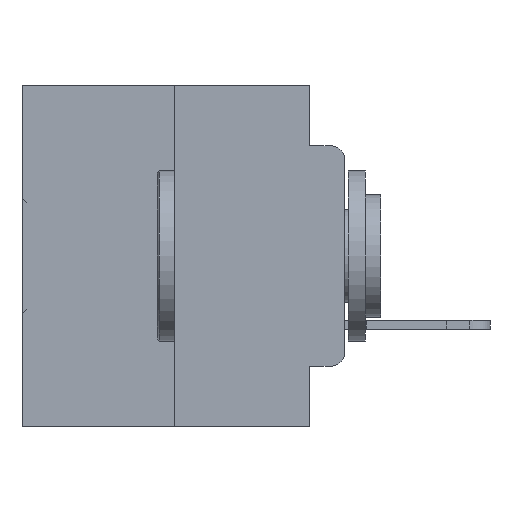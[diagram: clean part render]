
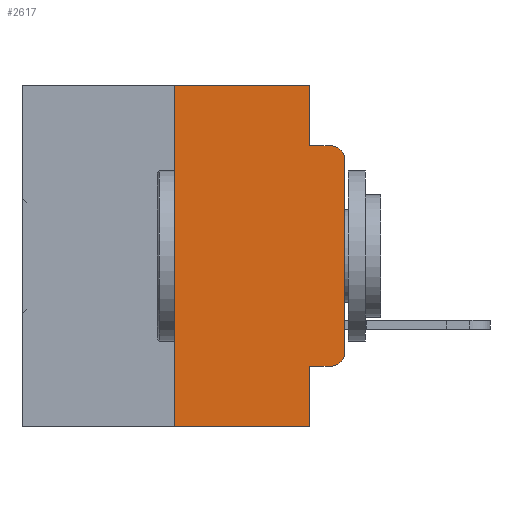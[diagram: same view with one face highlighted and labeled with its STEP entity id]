
A CAD part, left-side view. The second image highlights one B-rep face of the part: STEP entity #2617.
In plain terms, the highlighted planar face has unit normal (-1, 0, 0).
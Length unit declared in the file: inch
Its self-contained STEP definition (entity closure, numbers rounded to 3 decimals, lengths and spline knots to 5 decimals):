
#250 = ORIENTED_EDGE ( 'NONE', *, *, #6677, .T. ) ;
#1705 = CARTESIAN_POINT ( 'NONE',  ( 0., 0.051, -0.4115 ) ) ;
#1734 = ORIENTED_EDGE ( 'NONE', *, *, #12036, .F. ) ;
#1771 = LINE ( 'NONE', #17160, #15361 ) ;
#1961 = ORIENTED_EDGE ( 'NONE', *, *, #12135, .T. ) ;
#2097 = ORIENTED_EDGE ( 'NONE', *, *, #12140, .T. ) ;
#2617 = ADVANCED_FACE ( 'NONE', ( #4248 ), #13347, .F. ) ;
#4248 = FACE_OUTER_BOUND ( 'NONE', #5648, .T. ) ;
#5395 = VERTEX_POINT ( 'NONE', #32085 ) ;
#5648 = EDGE_LOOP ( 'NONE', ( #19901, #22186, #23280, #25613, #26177, #27823, #250, #1734, #1961, #2097 ) ) ;
#6668 = EDGE_CURVE ( 'NONE', #33246, #11114, #23879, .T. ) ;
#6677 = EDGE_CURVE ( 'NONE', #12878, #30754, #23019, .T. ) ;
#6907 = DIRECTION ( 'NONE',  ( 0., 0., -1. ) ) ;
#6994 = LINE ( 'NONE', #1705, #20261 ) ;
#7294 = CARTESIAN_POINT ( 'NONE',  ( 0., 0.02, -0.0885 ) ) ;
#7665 = CARTESIAN_POINT ( 'NONE',  ( 0., 0.051, 0. ) ) ;
#8056 = AXIS2_PLACEMENT_3D ( 'NONE', #18046, #33623, #17933 ) ;
#8332 = LINE ( 'NONE', #16361, #21516 ) ;
#9598 = VECTOR ( 'NONE', #6907, 39.37008 ) ;
#10053 = CIRCLE ( 'NONE', #8056, 0.02 ) ;
#10061 = VERTEX_POINT ( 'NONE', #12943 ) ;
#10124 = VERTEX_POINT ( 'NONE', #7294 ) ;
#10225 = DIRECTION ( 'NONE',  ( 0., 0., 1. ) ) ;
#11114 = VERTEX_POINT ( 'NONE', #12263 ) ;
#11682 = VECTOR ( 'NONE', #22231, 39.37008 ) ;
#11764 = EDGE_CURVE ( 'NONE', #33010, #33686, #32170, .T. ) ;
#11826 = EDGE_CURVE ( 'NONE', #33686, #10124, #10053, .T. ) ;
#11878 = EDGE_CURVE ( 'NONE', #10061, #10124, #1771, .T. ) ;
#11889 = EDGE_CURVE ( 'NONE', #11114, #10061, #8332, .T. ) ;
#11980 = EDGE_CURVE ( 'NONE', #12878, #33246, #26051, .T. ) ;
#12036 = EDGE_CURVE ( 'NONE', #5395, #30754, #17476, .T. ) ;
#12135 = EDGE_CURVE ( 'NONE', #5395, #19540, #6994, .T. ) ;
#12140 = EDGE_CURVE ( 'NONE', #19540, #33010, #27279, .T. ) ;
#12263 = CARTESIAN_POINT ( 'NONE',  ( 0., 0.051, 0. ) ) ;
#12878 = VERTEX_POINT ( 'NONE', #17045 ) ;
#12943 = CARTESIAN_POINT ( 'NONE',  ( 0., 0.051, -0.0885 ) ) ;
#13347 = PLANE ( 'NONE',  #20053 ) ;
#13898 = CARTESIAN_POINT ( 'NONE',  ( 0., 0.473, 0. ) ) ;
#14811 = DIRECTION ( 'NONE',  ( 0., 0., -1. ) ) ;
#14816 = DIRECTION ( 'NONE',  ( 1., 0., 0. ) ) ;
#15361 = VECTOR ( 'NONE', #16484, 39.37008 ) ;
#16122 = VECTOR ( 'NONE', #25430, 39.37008 ) ;
#16361 = CARTESIAN_POINT ( 'NONE',  ( 0., 0.051, 0. ) ) ;
#16484 = DIRECTION ( 'NONE',  ( 0., -1., 0. ) ) ;
#16923 = DIRECTION ( 'NONE',  ( 0., 0., -1. ) ) ;
#17045 = CARTESIAN_POINT ( 'NONE',  ( 0., 0.25, -0.5 ) ) ;
#17160 = CARTESIAN_POINT ( 'NONE',  ( 0., 0.051, -0.0885 ) ) ;
#17476 = LINE ( 'NONE', #7665, #9598 ) ;
#17933 = DIRECTION ( 'NONE',  ( 0., 0., -1. ) ) ;
#18046 = CARTESIAN_POINT ( 'NONE',  ( 0., 0.02, -0.1085 ) ) ;
#18738 = CARTESIAN_POINT ( 'NONE',  ( 0., 0.25, 0. ) ) ;
#19068 = VECTOR ( 'NONE', #10225, 39.37008 ) ;
#19537 = CARTESIAN_POINT ( 'NONE',  ( 0., 0.25, 0. ) ) ;
#19540 = VERTEX_POINT ( 'NONE', #28643 ) ;
#19901 = ORIENTED_EDGE ( 'NONE', *, *, #11764, .T. ) ;
#20053 = AXIS2_PLACEMENT_3D ( 'NONE', #13898, #14816, #14811 ) ;
#20261 = VECTOR ( 'NONE', #33410, 39.37008 ) ;
#21516 = VECTOR ( 'NONE', #16923, 39.37008 ) ;
#21771 = CARTESIAN_POINT ( 'NONE',  ( 0., 0., 0. ) ) ;
#22186 = ORIENTED_EDGE ( 'NONE', *, *, #11826, .T. ) ;
#22231 = DIRECTION ( 'NONE',  ( 0., 0., 1. ) ) ;
#23019 = LINE ( 'NONE', #25886, #16122 ) ;
#23280 = ORIENTED_EDGE ( 'NONE', *, *, #11878, .F. ) ;
#23628 = CARTESIAN_POINT ( 'NONE',  ( 0., 0.051, -0.5 ) ) ;
#23879 = LINE ( 'NONE', #26149, #25547 ) ;
#25430 = DIRECTION ( 'NONE',  ( 0., -1., 0. ) ) ;
#25547 = VECTOR ( 'NONE', #26638, 39.37008 ) ;
#25613 = ORIENTED_EDGE ( 'NONE', *, *, #11889, .F. ) ;
#25886 = CARTESIAN_POINT ( 'NONE',  ( 0., 0.473, -0.5 ) ) ;
#26051 = LINE ( 'NONE', #18738, #19068 ) ;
#26149 = CARTESIAN_POINT ( 'NONE',  ( 0., 0.473, 0. ) ) ;
#26177 = ORIENTED_EDGE ( 'NONE', *, *, #6668, .F. ) ;
#26637 = CARTESIAN_POINT ( 'NONE',  ( 0., 0., -0.1085 ) ) ;
#26638 = DIRECTION ( 'NONE',  ( 0., -1., 0. ) ) ;
#27279 = CIRCLE ( 'NONE', #33847, 0.02 ) ;
#27823 = ORIENTED_EDGE ( 'NONE', *, *, #11980, .F. ) ;
#28643 = CARTESIAN_POINT ( 'NONE',  ( 0., 0.02, -0.4115 ) ) ;
#30754 = VERTEX_POINT ( 'NONE', #23628 ) ;
#31174 = CARTESIAN_POINT ( 'NONE',  ( 0., 0., -0.3915 ) ) ;
#32085 = CARTESIAN_POINT ( 'NONE',  ( 0., 0.051, -0.4115 ) ) ;
#32170 = LINE ( 'NONE', #21771, #11682 ) ;
#33010 = VERTEX_POINT ( 'NONE', #31174 ) ;
#33122 = DIRECTION ( 'NONE',  ( 0., 0., -1. ) ) ;
#33146 = DIRECTION ( 'NONE',  ( -1., 0., 0. ) ) ;
#33209 = CARTESIAN_POINT ( 'NONE',  ( 0., 0.02, -0.3915 ) ) ;
#33246 = VERTEX_POINT ( 'NONE', #19537 ) ;
#33410 = DIRECTION ( 'NONE',  ( 0., -1., 0. ) ) ;
#33623 = DIRECTION ( 'NONE',  ( -1., 0., 0. ) ) ;
#33686 = VERTEX_POINT ( 'NONE', #26637 ) ;
#33847 = AXIS2_PLACEMENT_3D ( 'NONE', #33209, #33146, #33122 ) ;
